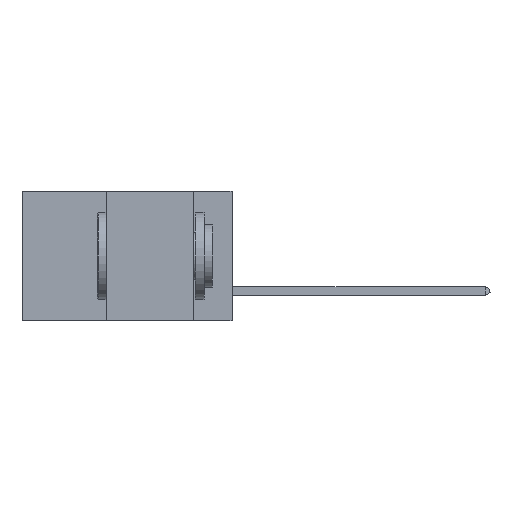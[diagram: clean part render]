
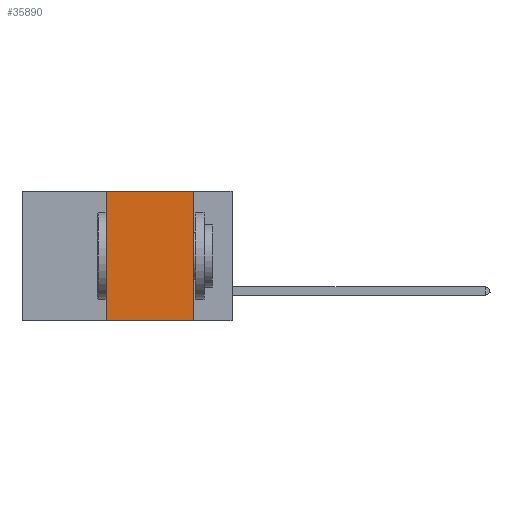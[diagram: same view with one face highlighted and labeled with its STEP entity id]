
A CAD part, left-side view. The second image highlights one B-rep face of the part: STEP entity #35890.
In plain terms, the highlighted planar face has unit normal (-1, 0, 0).
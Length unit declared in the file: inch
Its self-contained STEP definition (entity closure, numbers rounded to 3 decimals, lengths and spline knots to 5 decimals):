
#267 = CARTESIAN_POINT ( 'NONE',  ( 0., 0.36, 0. ) ) ;
#858 = CARTESIAN_POINT ( 'NONE',  ( 0., 0.11, 0. ) ) ;
#915 = EDGE_CURVE ( 'NONE', #36505, #3309, #32702, .T. ) ;
#1651 = VECTOR ( 'NONE', #33442, 39.37008 ) ;
#1863 = CARTESIAN_POINT ( 'NONE',  ( 0., 0.11, -0.37 ) ) ;
#3309 = VERTEX_POINT ( 'NONE', #1863 ) ;
#7078 = FACE_OUTER_BOUND ( 'NONE', #20551, .T. ) ;
#8643 = VECTOR ( 'NONE', #8834, 39.37008 ) ;
#8834 = DIRECTION ( 'NONE',  ( 0., -1., 0. ) ) ;
#10692 = ORIENTED_EDGE ( 'NONE', *, *, #28728, .T. ) ;
#12351 = ORIENTED_EDGE ( 'NONE', *, *, #32162, .F. ) ;
#14096 = CARTESIAN_POINT ( 'NONE',  ( 0., 0.36, 0. ) ) ;
#15451 = VECTOR ( 'NONE', #31556, 39.37008 ) ;
#16153 = DIRECTION ( 'NONE',  ( 0., 0., 1. ) ) ;
#19328 = DIRECTION ( 'NONE',  ( 0., 0., -1. ) ) ;
#20551 = EDGE_LOOP ( 'NONE', ( #33684, #12351, #29534, #10692 ) ) ;
#20554 = AXIS2_PLACEMENT_3D ( 'NONE', #28844, #31906, #19328 ) ;
#23724 = LINE ( 'NONE', #267, #34249 ) ;
#25566 = CARTESIAN_POINT ( 'NONE',  ( 0., 0.36, -0.37 ) ) ;
#27288 = VERTEX_POINT ( 'NONE', #25566 ) ;
#28495 = CARTESIAN_POINT ( 'NONE',  ( 0., 0.6, 0. ) ) ;
#28728 = EDGE_CURVE ( 'NONE', #27288, #3309, #31058, .T. ) ;
#28844 = CARTESIAN_POINT ( 'NONE',  ( 0., 0.6, 0. ) ) ;
#29534 = ORIENTED_EDGE ( 'NONE', *, *, #30276, .F. ) ;
#30026 = CARTESIAN_POINT ( 'NONE',  ( 0., 0.6, -0.37 ) ) ;
#30276 = EDGE_CURVE ( 'NONE', #27288, #38236, #23724, .T. ) ;
#31058 = LINE ( 'NONE', #30026, #8643 ) ;
#31508 = PLANE ( 'NONE',  #20554 ) ;
#31556 = DIRECTION ( 'NONE',  ( 0., -1., 0. ) ) ;
#31906 = DIRECTION ( 'NONE',  ( 1., 0., 0. ) ) ;
#32162 = EDGE_CURVE ( 'NONE', #38236, #36505, #32630, .T. ) ;
#32630 = LINE ( 'NONE', #28495, #15451 ) ;
#32702 = LINE ( 'NONE', #35995, #1651 ) ;
#33442 = DIRECTION ( 'NONE',  ( 0., 0., -1. ) ) ;
#33684 = ORIENTED_EDGE ( 'NONE', *, *, #915, .F. ) ;
#34249 = VECTOR ( 'NONE', #16153, 39.37008 ) ;
#35890 = ADVANCED_FACE ( 'NONE', ( #7078 ), #31508, .F. ) ;
#35995 = CARTESIAN_POINT ( 'NONE',  ( 0., 0.11, 0. ) ) ;
#36505 = VERTEX_POINT ( 'NONE', #858 ) ;
#38236 = VERTEX_POINT ( 'NONE', #14096 ) ;
